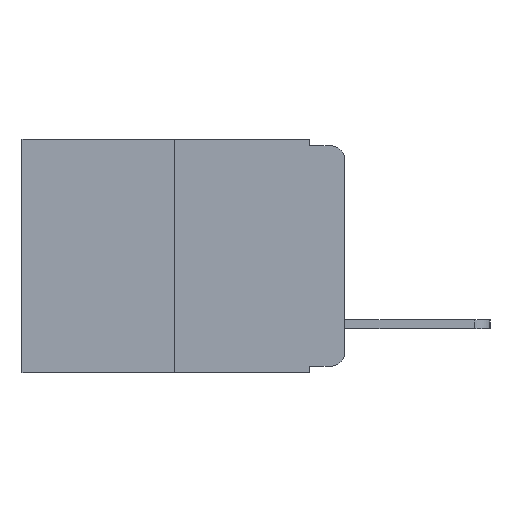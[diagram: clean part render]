
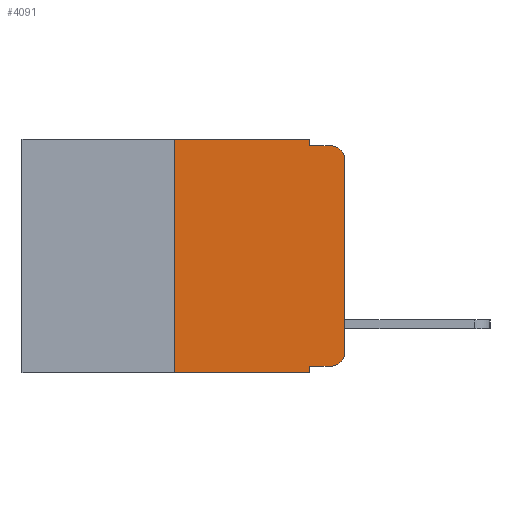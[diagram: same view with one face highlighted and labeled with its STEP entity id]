
A CAD part, left-side view. The second image highlights one B-rep face of the part: STEP entity #4091.
In plain terms, the highlighted planar face has unit normal (-1, 0, 0).
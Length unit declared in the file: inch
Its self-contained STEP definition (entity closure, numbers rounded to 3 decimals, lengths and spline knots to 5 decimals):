
#159 = EDGE_CURVE ( 'NONE', #11394, #5386, #2386, .T. ) ;
#179 = ORIENTED_EDGE ( 'NONE', *, *, #1559, .F. ) ;
#372 = DIRECTION ( 'NONE',  ( 0., -1., 0. ) ) ;
#426 = CARTESIAN_POINT ( 'NONE',  ( 0., 0., -0.313 ) ) ;
#465 = CARTESIAN_POINT ( 'NONE',  ( 0., 0.051, 0. ) ) ;
#467 = EDGE_CURVE ( 'NONE', #7767, #6429, #2567, .T. ) ;
#473 = EDGE_CURVE ( 'NONE', #6429, #1373, #10976, .T. ) ;
#603 = DIRECTION ( 'NONE',  ( 0., -1., 0. ) ) ;
#647 = PLANE ( 'NONE',  #6324 ) ;
#737 = ORIENTED_EDGE ( 'NONE', *, *, #159, .T. ) ;
#746 = ORIENTED_EDGE ( 'NONE', *, *, #1593, .F. ) ;
#966 = CARTESIAN_POINT ( 'NONE',  ( 0., 0.02, -0.333 ) ) ;
#1068 = ORIENTED_EDGE ( 'NONE', *, *, #4080, .F. ) ;
#1126 = CARTESIAN_POINT ( 'NONE',  ( 0., 0.051, -0.333 ) ) ;
#1128 = EDGE_CURVE ( 'NONE', #3808, #1373, #7462, .T. ) ;
#1205 = ORIENTED_EDGE ( 'NONE', *, *, #1128, .F. ) ;
#1297 = CARTESIAN_POINT ( 'NONE',  ( 0., 0.02, -0.01 ) ) ;
#1314 = CARTESIAN_POINT ( 'NONE',  ( 0., 0.25, -0.343 ) ) ;
#1373 = VERTEX_POINT ( 'NONE', #1297 ) ;
#1543 = LINE ( 'NONE', #1126, #10465 ) ;
#1559 = EDGE_CURVE ( 'NONE', #2975, #3808, #8973, .T. ) ;
#1593 = EDGE_CURVE ( 'NONE', #11394, #1647, #4176, .T. ) ;
#1633 = DIRECTION ( 'NONE',  ( 1., 0., 0. ) ) ;
#1647 = VERTEX_POINT ( 'NONE', #2968 ) ;
#1830 = EDGE_CURVE ( 'NONE', #1834, #5386, #3036, .T. ) ;
#1834 = VERTEX_POINT ( 'NONE', #6708 ) ;
#2025 = EDGE_CURVE ( 'NONE', #1834, #9375, #1543, .T. ) ;
#2050 = EDGE_CURVE ( 'NONE', #9375, #7767, #5875, .T. ) ;
#2159 = ORIENTED_EDGE ( 'NONE', *, *, #2025, .T. ) ;
#2386 = LINE ( 'NONE', #10218, #9248 ) ;
#2548 = VECTOR ( 'NONE', #2742, 39.37008 ) ;
#2567 = LINE ( 'NONE', #4409, #4659 ) ;
#2654 = CARTESIAN_POINT ( 'NONE',  ( 0., 0.473, 0. ) ) ;
#2742 = DIRECTION ( 'NONE',  ( 0., -1., 0. ) ) ;
#2869 = LINE ( 'NONE', #8088, #9098 ) ;
#2968 = CARTESIAN_POINT ( 'NONE',  ( 0., 0.25, 0. ) ) ;
#2975 = VERTEX_POINT ( 'NONE', #4704 ) ;
#3036 = LINE ( 'NONE', #465, #9980 ) ;
#3043 = ORIENTED_EDGE ( 'NONE', *, *, #473, .T. ) ;
#3274 = ORIENTED_EDGE ( 'NONE', *, *, #467, .T. ) ;
#3808 = VERTEX_POINT ( 'NONE', #4766 ) ;
#4080 = EDGE_CURVE ( 'NONE', #1647, #2975, #2869, .T. ) ;
#4091 = ADVANCED_FACE ( 'NONE', ( #6941 ), #647, .F. ) ;
#4176 = LINE ( 'NONE', #10956, #6302 ) ;
#4409 = CARTESIAN_POINT ( 'NONE',  ( 0., 0., 0. ) ) ;
#4491 = VECTOR ( 'NONE', #11116, 39.37008 ) ;
#4659 = VECTOR ( 'NONE', #7773, 39.37008 ) ;
#4704 = CARTESIAN_POINT ( 'NONE',  ( 0., 0.051, 0. ) ) ;
#4766 = CARTESIAN_POINT ( 'NONE',  ( 0., 0.051, -0.01 ) ) ;
#5190 = DIRECTION ( 'NONE',  ( 0., 0., -1. ) ) ;
#5386 = VERTEX_POINT ( 'NONE', #8904 ) ;
#5390 = ORIENTED_EDGE ( 'NONE', *, *, #1830, .F. ) ;
#5555 = DIRECTION ( 'NONE',  ( 0., -1., 0. ) ) ;
#5734 = ORIENTED_EDGE ( 'NONE', *, *, #2050, .T. ) ;
#5875 = CIRCLE ( 'NONE', #8939, 0.02 ) ;
#6015 = CARTESIAN_POINT ( 'NONE',  ( 0., 0.051, -0.01 ) ) ;
#6302 = VECTOR ( 'NONE', #7847, 39.37008 ) ;
#6324 = AXIS2_PLACEMENT_3D ( 'NONE', #2654, #1633, #8131 ) ;
#6429 = VERTEX_POINT ( 'NONE', #6785 ) ;
#6595 = CARTESIAN_POINT ( 'NONE',  ( 0., 0.02, -0.313 ) ) ;
#6708 = CARTESIAN_POINT ( 'NONE',  ( 0., 0.051, -0.333 ) ) ;
#6785 = CARTESIAN_POINT ( 'NONE',  ( 0., 0., -0.03 ) ) ;
#6941 = FACE_OUTER_BOUND ( 'NONE', #7578, .T. ) ;
#7441 = CARTESIAN_POINT ( 'NONE',  ( 0., 0.02, -0.03 ) ) ;
#7462 = LINE ( 'NONE', #6015, #2548 ) ;
#7578 = EDGE_LOOP ( 'NONE', ( #3274, #3043, #1205, #179, #1068, #746, #737, #5390, #2159, #5734 ) ) ;
#7595 = DIRECTION ( 'NONE',  ( -1., 0., 0. ) ) ;
#7767 = VERTEX_POINT ( 'NONE', #426 ) ;
#7773 = DIRECTION ( 'NONE',  ( 0., 0., 1. ) ) ;
#7828 = DIRECTION ( 'NONE',  ( 0., 0., -1. ) ) ;
#7847 = DIRECTION ( 'NONE',  ( 0., 0., 1. ) ) ;
#8088 = CARTESIAN_POINT ( 'NONE',  ( 0., 0.473, 0. ) ) ;
#8131 = DIRECTION ( 'NONE',  ( 0., 0., -1. ) ) ;
#8263 = DIRECTION ( 'NONE',  ( 0., 0., -1. ) ) ;
#8523 = AXIS2_PLACEMENT_3D ( 'NONE', #7441, #7595, #7828 ) ;
#8904 = CARTESIAN_POINT ( 'NONE',  ( 0., 0.051, -0.343 ) ) ;
#8939 = AXIS2_PLACEMENT_3D ( 'NONE', #6595, #11483, #8263 ) ;
#8973 = LINE ( 'NONE', #10435, #4491 ) ;
#9098 = VECTOR ( 'NONE', #603, 39.37008 ) ;
#9248 = VECTOR ( 'NONE', #5555, 39.37008 ) ;
#9375 = VERTEX_POINT ( 'NONE', #966 ) ;
#9980 = VECTOR ( 'NONE', #5190, 39.37008 ) ;
#10218 = CARTESIAN_POINT ( 'NONE',  ( 0., 0.473, -0.343 ) ) ;
#10435 = CARTESIAN_POINT ( 'NONE',  ( 0., 0.051, 0. ) ) ;
#10465 = VECTOR ( 'NONE', #372, 39.37008 ) ;
#10956 = CARTESIAN_POINT ( 'NONE',  ( 0., 0.25, 0. ) ) ;
#10976 = CIRCLE ( 'NONE', #8523, 0.02 ) ;
#11116 = DIRECTION ( 'NONE',  ( 0., 0., -1. ) ) ;
#11394 = VERTEX_POINT ( 'NONE', #1314 ) ;
#11483 = DIRECTION ( 'NONE',  ( -1., 0., 0. ) ) ;
